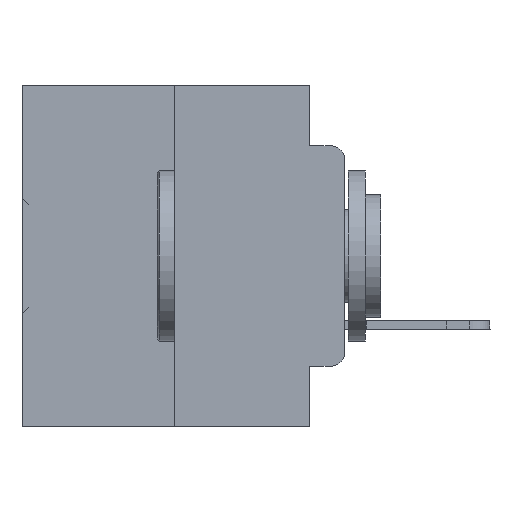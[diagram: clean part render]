
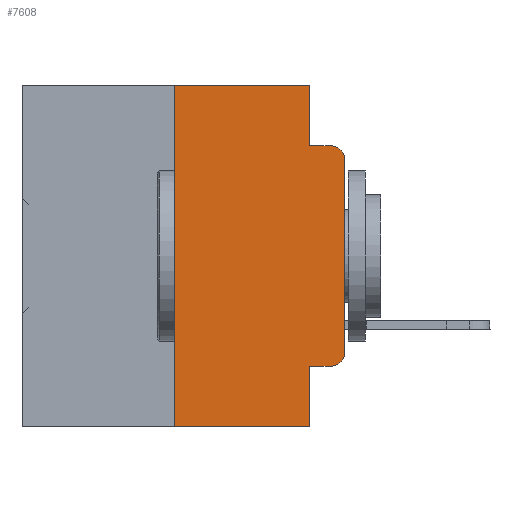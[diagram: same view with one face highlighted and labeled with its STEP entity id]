
A CAD part, left-side view. The second image highlights one B-rep face of the part: STEP entity #7608.
In plain terms, the highlighted planar face has unit normal (-1, 0, 0).
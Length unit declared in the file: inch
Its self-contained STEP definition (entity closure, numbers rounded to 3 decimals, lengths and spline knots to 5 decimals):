
#144 = DIRECTION ( 'NONE',  ( 0., -1., 0. ) ) ;
#302 = VECTOR ( 'NONE', #29491, 39.37008 ) ;
#1015 = DIRECTION ( 'NONE',  ( 0., 0., -1. ) ) ;
#1057 = ORIENTED_EDGE ( 'NONE', *, *, #29793, .F. ) ;
#1911 = EDGE_CURVE ( 'NONE', #23339, #34573, #2268, .T. ) ;
#2094 = EDGE_CURVE ( 'NONE', #6908, #15527, #20843, .T. ) ;
#2268 = LINE ( 'NONE', #7839, #14469 ) ;
#2481 = FACE_OUTER_BOUND ( 'NONE', #28308, .T. ) ;
#3479 = CARTESIAN_POINT ( 'NONE',  ( 0., 0.473, -0.5 ) ) ;
#4544 = ORIENTED_EDGE ( 'NONE', *, *, #31693, .T. ) ;
#4781 = EDGE_CURVE ( 'NONE', #37776, #6908, #19373, .T. ) ;
#5356 = DIRECTION ( 'NONE',  ( 1., 0., 0. ) ) ;
#5358 = DIRECTION ( 'NONE',  ( 0., -1., 0. ) ) ;
#6326 = CARTESIAN_POINT ( 'NONE',  ( 0., 0.02, -0.1085 ) ) ;
#6908 = VERTEX_POINT ( 'NONE', #8765 ) ;
#7608 = ADVANCED_FACE ( 'NONE', ( #2481 ), #16463, .F. ) ;
#7839 = CARTESIAN_POINT ( 'NONE',  ( 0., 0.25, 0. ) ) ;
#8629 = CARTESIAN_POINT ( 'NONE',  ( 0., 0.051, -0.4115 ) ) ;
#8765 = CARTESIAN_POINT ( 'NONE',  ( 0., 0.051, -0.0885 ) ) ;
#9253 = LINE ( 'NONE', #3479, #35292 ) ;
#9633 = LINE ( 'NONE', #15540, #34901 ) ;
#9650 = VERTEX_POINT ( 'NONE', #21983 ) ;
#9655 = CARTESIAN_POINT ( 'NONE',  ( 0., 0.051, 0. ) ) ;
#9945 = CIRCLE ( 'NONE', #29461, 0.02 ) ;
#10730 = DIRECTION ( 'NONE',  ( 0., 0., 1. ) ) ;
#10781 = CARTESIAN_POINT ( 'NONE',  ( 0., 0.051, 0. ) ) ;
#11409 = ORIENTED_EDGE ( 'NONE', *, *, #13668, .T. ) ;
#11651 = VECTOR ( 'NONE', #18653, 39.37008 ) ;
#13518 = CARTESIAN_POINT ( 'NONE',  ( 0., 0., -0.1085 ) ) ;
#13668 = EDGE_CURVE ( 'NONE', #23339, #28070, #9253, .T. ) ;
#14309 = ORIENTED_EDGE ( 'NONE', *, *, #21631, .F. ) ;
#14469 = VECTOR ( 'NONE', #10730, 39.37008 ) ;
#14692 = CARTESIAN_POINT ( 'NONE',  ( 0., 0.02, -0.4115 ) ) ;
#15036 = ORIENTED_EDGE ( 'NONE', *, *, #4781, .F. ) ;
#15217 = CARTESIAN_POINT ( 'NONE',  ( 0., 0., 0. ) ) ;
#15527 = VERTEX_POINT ( 'NONE', #27744 ) ;
#15540 = CARTESIAN_POINT ( 'NONE',  ( 0., 0.473, 0. ) ) ;
#15909 = DIRECTION ( 'NONE',  ( 0., -1., 0. ) ) ;
#16463 = PLANE ( 'NONE',  #20822 ) ;
#16887 = VECTOR ( 'NONE', #144, 39.37008 ) ;
#17097 = VERTEX_POINT ( 'NONE', #25762 ) ;
#18188 = DIRECTION ( 'NONE',  ( -1., 0., 0. ) ) ;
#18562 = DIRECTION ( 'NONE',  ( 0., 0., -1. ) ) ;
#18653 = DIRECTION ( 'NONE',  ( 0., 0., 1. ) ) ;
#18657 = DIRECTION ( 'NONE',  ( 0., 0., -1. ) ) ;
#19373 = LINE ( 'NONE', #10781, #302 ) ;
#20021 = VECTOR ( 'NONE', #5358, 39.37008 ) ;
#20822 = AXIS2_PLACEMENT_3D ( 'NONE', #28721, #5356, #31199 ) ;
#20843 = LINE ( 'NONE', #26404, #16887 ) ;
#21109 = DIRECTION ( 'NONE',  ( 0., -1., 0. ) ) ;
#21236 = EDGE_CURVE ( 'NONE', #17097, #31959, #36077, .T. ) ;
#21631 = EDGE_CURVE ( 'NONE', #34573, #37776, #9633, .T. ) ;
#21857 = ORIENTED_EDGE ( 'NONE', *, *, #23279, .T. ) ;
#21983 = CARTESIAN_POINT ( 'NONE',  ( 0., 0.051, -0.4115 ) ) ;
#22062 = CARTESIAN_POINT ( 'NONE',  ( 0., 0.051, -0.5 ) ) ;
#22520 = EDGE_CURVE ( 'NONE', #30452, #17097, #9945, .T. ) ;
#23279 = EDGE_CURVE ( 'NONE', #31959, #15527, #33182, .T. ) ;
#23339 = VERTEX_POINT ( 'NONE', #32552 ) ;
#24605 = ORIENTED_EDGE ( 'NONE', *, *, #1911, .F. ) ;
#25489 = ORIENTED_EDGE ( 'NONE', *, *, #21236, .T. ) ;
#25762 = CARTESIAN_POINT ( 'NONE',  ( 0., 0., -0.3915 ) ) ;
#26404 = CARTESIAN_POINT ( 'NONE',  ( 0., 0.051, -0.0885 ) ) ;
#26474 = AXIS2_PLACEMENT_3D ( 'NONE', #6326, #18188, #18562 ) ;
#27249 = LINE ( 'NONE', #9655, #36417 ) ;
#27744 = CARTESIAN_POINT ( 'NONE',  ( 0., 0.02, -0.0885 ) ) ;
#28070 = VERTEX_POINT ( 'NONE', #22062 ) ;
#28308 = EDGE_LOOP ( 'NONE', ( #25489, #21857, #29431, #15036, #14309, #24605, #11409, #1057, #4544, #29192 ) ) ;
#28721 = CARTESIAN_POINT ( 'NONE',  ( 0., 0.473, 0. ) ) ;
#29192 = ORIENTED_EDGE ( 'NONE', *, *, #22520, .T. ) ;
#29431 = ORIENTED_EDGE ( 'NONE', *, *, #2094, .F. ) ;
#29461 = AXIS2_PLACEMENT_3D ( 'NONE', #32507, #36456, #18657 ) ;
#29491 = DIRECTION ( 'NONE',  ( 0., 0., -1. ) ) ;
#29793 = EDGE_CURVE ( 'NONE', #9650, #28070, #27249, .T. ) ;
#30452 = VERTEX_POINT ( 'NONE', #14692 ) ;
#31199 = DIRECTION ( 'NONE',  ( 0., 0., -1. ) ) ;
#31693 = EDGE_CURVE ( 'NONE', #9650, #30452, #31783, .T. ) ;
#31783 = LINE ( 'NONE', #8629, #20021 ) ;
#31959 = VERTEX_POINT ( 'NONE', #13518 ) ;
#32507 = CARTESIAN_POINT ( 'NONE',  ( 0., 0.02, -0.3915 ) ) ;
#32552 = CARTESIAN_POINT ( 'NONE',  ( 0., 0.25, -0.5 ) ) ;
#33182 = CIRCLE ( 'NONE', #26474, 0.02 ) ;
#33671 = CARTESIAN_POINT ( 'NONE',  ( 0., 0.051, 0. ) ) ;
#34573 = VERTEX_POINT ( 'NONE', #36191 ) ;
#34901 = VECTOR ( 'NONE', #21109, 39.37008 ) ;
#35292 = VECTOR ( 'NONE', #15909, 39.37008 ) ;
#36077 = LINE ( 'NONE', #15217, #11651 ) ;
#36191 = CARTESIAN_POINT ( 'NONE',  ( 0., 0.25, 0. ) ) ;
#36417 = VECTOR ( 'NONE', #1015, 39.37008 ) ;
#36456 = DIRECTION ( 'NONE',  ( -1., 0., 0. ) ) ;
#37776 = VERTEX_POINT ( 'NONE', #33671 ) ;
